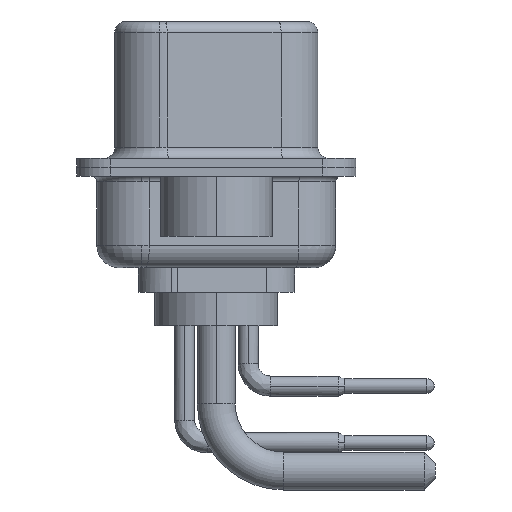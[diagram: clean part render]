
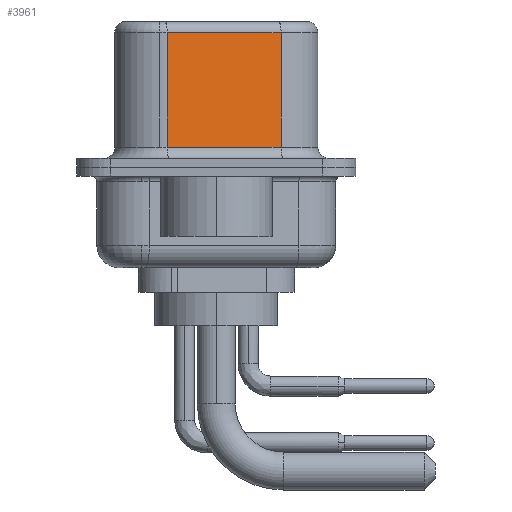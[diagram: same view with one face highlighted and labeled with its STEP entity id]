
A CAD part, left-side view. The second image highlights one B-rep face of the part: STEP entity #3961.
In plain terms, the highlighted planar face has unit normal (-0.985, -0.174, 0).
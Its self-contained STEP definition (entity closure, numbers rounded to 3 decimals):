
#193 = EDGE_CURVE ( 'NONE', #10398, #16145, #15151, .T. ) ;
#452 = CARTESIAN_POINT ( 'NONE',  ( 3.68, 2.203, 6.52 ) ) ;
#3961 = ADVANCED_FACE ( 'NONE', ( #17964 ), #12190, .F. ) ;
#4998 = CARTESIAN_POINT ( 'NONE',  ( 4.58, -2.897, 6.02 ) ) ;
#6116 = VERTEX_POINT ( 'NONE', #23577 ) ;
#6341 = CARTESIAN_POINT ( 'NONE',  ( 4.58, -2.897, 0.9 ) ) ;
#6990 = ORIENTED_EDGE ( 'NONE', *, *, #15445, .T. ) ;
#7015 = CARTESIAN_POINT ( 'NONE',  ( 4.58, -2.897, 0.9 ) ) ;
#7748 = CARTESIAN_POINT ( 'NONE',  ( 3.68, 2.203, 0.9 ) ) ;
#8541 = DIRECTION ( 'NONE',  ( 0.985, 0.174, 0. ) ) ;
#8751 = EDGE_CURVE ( 'NONE', #6116, #22829, #23795, .T. ) ;
#9116 = VECTOR ( 'NONE', #13862, 1000. ) ;
#9755 = VECTOR ( 'NONE', #23552, 1000. ) ;
#10398 = VERTEX_POINT ( 'NONE', #7748 ) ;
#10510 = DIRECTION ( 'NONE',  ( 0., 0., -1. ) ) ;
#10667 = CARTESIAN_POINT ( 'NONE',  ( 4.58, -2.897, 6.52 ) ) ;
#11764 = AXIS2_PLACEMENT_3D ( 'NONE', #10667, #8541, #12426 ) ;
#12009 = EDGE_CURVE ( 'NONE', #6116, #16145, #15257, .T. ) ;
#12190 = PLANE ( 'NONE',  #11764 ) ;
#12426 = DIRECTION ( 'NONE',  ( -0.174, 0.985, 0. ) ) ;
#12825 = ORIENTED_EDGE ( 'NONE', *, *, #193, .T. ) ;
#13552 = ORIENTED_EDGE ( 'NONE', *, *, #8751, .T. ) ;
#13862 = DIRECTION ( 'NONE',  ( 0., 0., -1. ) ) ;
#15151 = LINE ( 'NONE', #6341, #19297 ) ;
#15257 = LINE ( 'NONE', #22655, #18656 ) ;
#15445 = EDGE_CURVE ( 'NONE', #22829, #10398, #17641, .T. ) ;
#15498 = EDGE_LOOP ( 'NONE', ( #21373, #13552, #6990, #12825 ) ) ;
#16145 = VERTEX_POINT ( 'NONE', #7015 ) ;
#17641 = LINE ( 'NONE', #452, #9116 ) ;
#17964 = FACE_OUTER_BOUND ( 'NONE', #15498, .T. ) ;
#18656 = VECTOR ( 'NONE', #10510, 1000. ) ;
#19297 = VECTOR ( 'NONE', #21266, 1000. ) ;
#21266 = DIRECTION ( 'NONE',  ( 0.174, -0.985, 0. ) ) ;
#21373 = ORIENTED_EDGE ( 'NONE', *, *, #12009, .F. ) ;
#21982 = CARTESIAN_POINT ( 'NONE',  ( 3.68, 2.203, 6.02 ) ) ;
#22655 = CARTESIAN_POINT ( 'NONE',  ( 4.58, -2.897, 6.52 ) ) ;
#22829 = VERTEX_POINT ( 'NONE', #21982 ) ;
#23552 = DIRECTION ( 'NONE',  ( -0.174, 0.985, 0. ) ) ;
#23577 = CARTESIAN_POINT ( 'NONE',  ( 4.58, -2.897, 6.02 ) ) ;
#23795 = LINE ( 'NONE', #4998, #9755 ) ;
